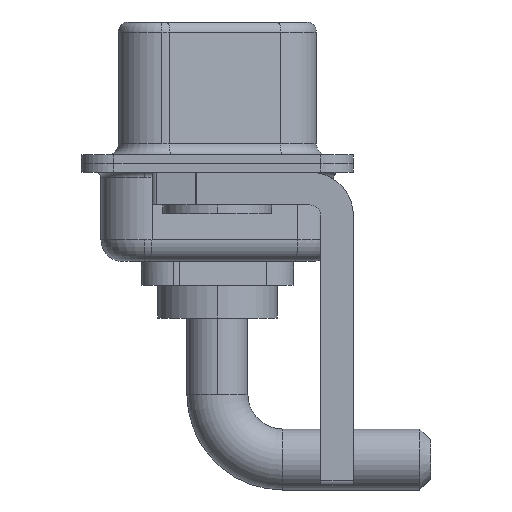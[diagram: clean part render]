
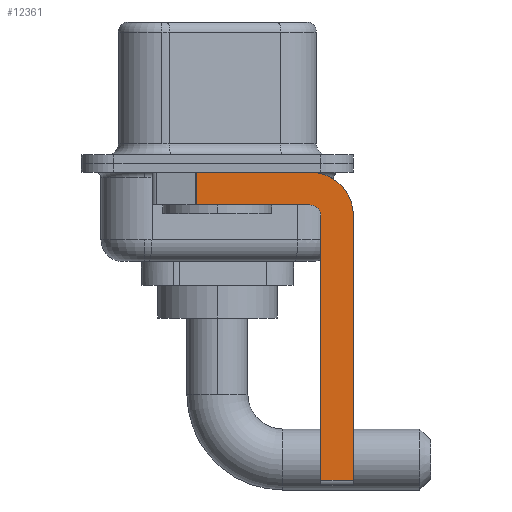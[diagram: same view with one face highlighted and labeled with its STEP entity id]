
A CAD part, left-side view. The second image highlights one B-rep face of the part: STEP entity #12361.
In plain terms, the highlighted planar face has unit normal (-1, 0, 0).
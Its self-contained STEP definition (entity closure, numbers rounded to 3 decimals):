
#98 = VERTEX_POINT ( 'NONE', #2850 ) ;
#125 = VERTEX_POINT ( 'NONE', #13571 ) ;
#1126 = EDGE_CURVE ( 'NONE', #11073, #8879, #6715, .T. ) ;
#1501 = CARTESIAN_POINT ( 'NONE',  ( -2.9, 0.978, -1.9 ) ) ;
#1559 = DIRECTION ( 'NONE',  ( 0., 1., 0. ) ) ;
#1753 = EDGE_CURVE ( 'NONE', #11073, #11354, #14625, .T. ) ;
#2168 = ORIENTED_EDGE ( 'NONE', *, *, #14170, .F. ) ;
#2232 = EDGE_CURVE ( 'NONE', #9860, #15152, #13241, .T. ) ;
#2510 = CARTESIAN_POINT ( 'NONE',  ( -2.9, -4.75, -2.4 ) ) ;
#2842 = VERTEX_POINT ( 'NONE', #14816 ) ;
#2850 = CARTESIAN_POINT ( 'NONE',  ( -2.9, -6.25, -14.55 ) ) ;
#3423 = VECTOR ( 'NONE', #1559, 1000. ) ;
#3627 = CARTESIAN_POINT ( 'NONE',  ( -2.9, -4.25, -1.9 ) ) ;
#3731 = CARTESIAN_POINT ( 'NONE',  ( -2.9, -4.25, -14.55 ) ) ;
#4080 = EDGE_CURVE ( 'NONE', #9860, #98, #9325, .T. ) ;
#4230 = DIRECTION ( 'NONE',  ( 0., 0., -1. ) ) ;
#4287 = DIRECTION ( 'NONE',  ( 0., 0., -1. ) ) ;
#4342 = VECTOR ( 'NONE', #6284, 1000. ) ;
#4364 = EDGE_CURVE ( 'NONE', #2842, #98, #8991, .T. ) ;
#4575 = VECTOR ( 'NONE', #6301, 1000. ) ;
#4800 = ORIENTED_EDGE ( 'NONE', *, *, #4364, .F. ) ;
#4872 = AXIS2_PLACEMENT_3D ( 'NONE', #7562, #12251, #8852 ) ;
#5362 = FACE_OUTER_BOUND ( 'NONE', #7566, .T. ) ;
#5528 = ORIENTED_EDGE ( 'NONE', *, *, #2232, .F. ) ;
#5951 = AXIS2_PLACEMENT_3D ( 'NONE', #9757, #13484, #4287 ) ;
#6197 = CIRCLE ( 'NONE', #5951, 2. ) ;
#6284 = DIRECTION ( 'NONE',  ( 0., 0., 1. ) ) ;
#6301 = DIRECTION ( 'NONE',  ( 0., 0., -1. ) ) ;
#6430 = VECTOR ( 'NONE', #11776, 1000. ) ;
#6715 = LINE ( 'NONE', #12603, #10744 ) ;
#6921 = CARTESIAN_POINT ( 'NONE',  ( -2.9, -4.25, -0.4 ) ) ;
#7562 = CARTESIAN_POINT ( 'NONE',  ( -2.9, -4.25, -2.4 ) ) ;
#7566 = EDGE_LOOP ( 'NONE', ( #12888, #8840, #12660, #15027, #5528, #10852, #4800, #2168 ) ) ;
#7688 = CARTESIAN_POINT ( 'NONE',  ( -2.9, -4.25, -2.4 ) ) ;
#7904 = VECTOR ( 'NONE', #14819, 1000. ) ;
#8840 = ORIENTED_EDGE ( 'NONE', *, *, #1753, .T. ) ;
#8852 = DIRECTION ( 'NONE',  ( 0., 0., 1. ) ) ;
#8879 = VERTEX_POINT ( 'NONE', #6921 ) ;
#8991 = LINE ( 'NONE', #11427, #7904 ) ;
#9325 = LINE ( 'NONE', #3731, #6430 ) ;
#9553 = CIRCLE ( 'NONE', #4872, 0.5 ) ;
#9757 = CARTESIAN_POINT ( 'NONE',  ( -2.9, -4.25, -2.4 ) ) ;
#9805 = EDGE_CURVE ( 'NONE', #15152, #125, #9553, .T. ) ;
#9860 = VERTEX_POINT ( 'NONE', #10312 ) ;
#10065 = PLANE ( 'NONE',  #11059 ) ;
#10312 = CARTESIAN_POINT ( 'NONE',  ( -2.9, -4.75, -14.55 ) ) ;
#10445 = EDGE_CURVE ( 'NONE', #125, #11354, #14201, .T. ) ;
#10744 = VECTOR ( 'NONE', #13523, 1000. ) ;
#10852 = ORIENTED_EDGE ( 'NONE', *, *, #4080, .T. ) ;
#11059 = AXIS2_PLACEMENT_3D ( 'NONE', #7688, #14738, #4230 ) ;
#11073 = VERTEX_POINT ( 'NONE', #13342 ) ;
#11095 = CARTESIAN_POINT ( 'NONE',  ( -2.9, 0.978, -1.9 ) ) ;
#11157 = CARTESIAN_POINT ( 'NONE',  ( -2.9, -4.75, -14.8 ) ) ;
#11354 = VERTEX_POINT ( 'NONE', #1501 ) ;
#11427 = CARTESIAN_POINT ( 'NONE',  ( -2.9, -6.25, -2.4 ) ) ;
#11776 = DIRECTION ( 'NONE',  ( 0., -1., 0. ) ) ;
#12251 = DIRECTION ( 'NONE',  ( -1., 0., 0. ) ) ;
#12361 = ADVANCED_FACE ( 'NONE', ( #5362 ), #10065, .F. ) ;
#12603 = CARTESIAN_POINT ( 'NONE',  ( -2.9, 3., -0.4 ) ) ;
#12660 = ORIENTED_EDGE ( 'NONE', *, *, #10445, .F. ) ;
#12888 = ORIENTED_EDGE ( 'NONE', *, *, #1126, .F. ) ;
#13241 = LINE ( 'NONE', #11157, #4342 ) ;
#13342 = CARTESIAN_POINT ( 'NONE',  ( -2.9, 0.978, -0.4 ) ) ;
#13484 = DIRECTION ( 'NONE',  ( 1., 0., 0. ) ) ;
#13523 = DIRECTION ( 'NONE',  ( 0., -1., 0. ) ) ;
#13571 = CARTESIAN_POINT ( 'NONE',  ( -2.9, -4.25, -1.9 ) ) ;
#14170 = EDGE_CURVE ( 'NONE', #8879, #2842, #6197, .T. ) ;
#14201 = LINE ( 'NONE', #3627, #3423 ) ;
#14625 = LINE ( 'NONE', #11095, #4575 ) ;
#14738 = DIRECTION ( 'NONE',  ( 1., 0., 0. ) ) ;
#14816 = CARTESIAN_POINT ( 'NONE',  ( -2.9, -6.25, -2.4 ) ) ;
#14819 = DIRECTION ( 'NONE',  ( 0., 0., -1. ) ) ;
#15027 = ORIENTED_EDGE ( 'NONE', *, *, #9805, .F. ) ;
#15152 = VERTEX_POINT ( 'NONE', #2510 ) ;
